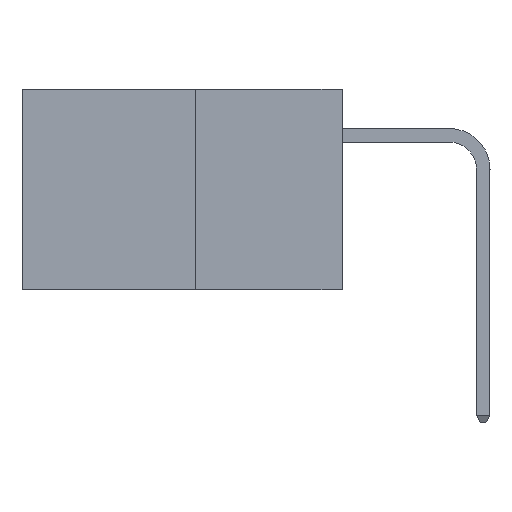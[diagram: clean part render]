
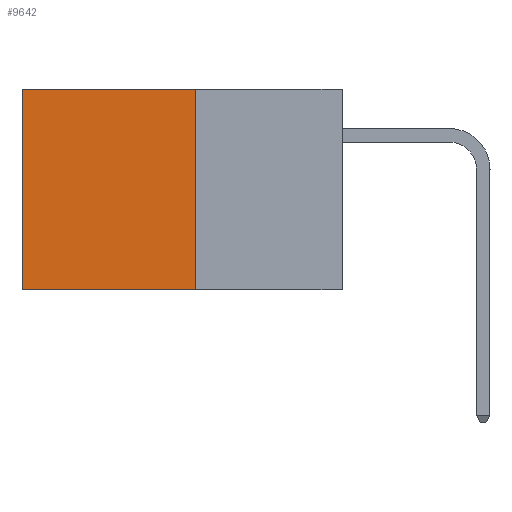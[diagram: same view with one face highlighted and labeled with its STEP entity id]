
A CAD part, left-side view. The second image highlights one B-rep face of the part: STEP entity #9642.
In plain terms, the highlighted planar face has unit normal (-1, 0, 0).
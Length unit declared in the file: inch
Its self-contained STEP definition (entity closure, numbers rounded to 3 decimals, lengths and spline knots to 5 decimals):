
#85 = CARTESIAN_POINT ( 'NONE',  ( 0.277, 0.27, 0. ) ) ;
#335 = DIRECTION ( 'NONE',  ( 0., 1., 0. ) ) ;
#445 = CARTESIAN_POINT ( 'NONE',  ( 0.277, 0.27, 0. ) ) ;
#870 = ORIENTED_EDGE ( 'NONE', *, *, #7032, .T. ) ;
#891 = CARTESIAN_POINT ( 'NONE',  ( 0.277, 0.27, -0.37 ) ) ;
#1509 = VECTOR ( 'NONE', #27543, 39.37008 ) ;
#1999 = AXIS2_PLACEMENT_3D ( 'NONE', #891, #3387, #20229 ) ;
#3387 = DIRECTION ( 'NONE',  ( 1., 0., 0. ) ) ;
#4537 = VECTOR ( 'NONE', #9559, 39.37008 ) ;
#5683 = ORIENTED_EDGE ( 'NONE', *, *, #7446, .F. ) ;
#6428 = VECTOR ( 'NONE', #335, 39.37008 ) ;
#7032 = EDGE_CURVE ( 'NONE', #19737, #27350, #27212, .T. ) ;
#7446 = EDGE_CURVE ( 'NONE', #8214, #23237, #7608, .T. ) ;
#7608 = LINE ( 'NONE', #17515, #13222 ) ;
#8106 = EDGE_CURVE ( 'NONE', #8214, #19737, #25670, .T. ) ;
#8214 = VERTEX_POINT ( 'NONE', #85 ) ;
#9559 = DIRECTION ( 'NONE',  ( 0., 1., 0. ) ) ;
#9642 = ADVANCED_FACE ( 'NONE', ( #23673 ), #15342, .F. ) ;
#13222 = VECTOR ( 'NONE', #17358, 39.37008 ) ;
#15241 = CARTESIAN_POINT ( 'NONE',  ( 0.277, 0.59, 0. ) ) ;
#15342 = PLANE ( 'NONE',  #1999 ) ;
#15514 = CARTESIAN_POINT ( 'NONE',  ( 0.277, 0.59, -0.37 ) ) ;
#17058 = ORIENTED_EDGE ( 'NONE', *, *, #23799, .F. ) ;
#17358 = DIRECTION ( 'NONE',  ( 0., 0., -1. ) ) ;
#17515 = CARTESIAN_POINT ( 'NONE',  ( 0.277, 0.27, -0.37 ) ) ;
#18848 = LINE ( 'NONE', #21587, #4537 ) ;
#19737 = VERTEX_POINT ( 'NONE', #15241 ) ;
#20229 = DIRECTION ( 'NONE',  ( 0., 0., -1. ) ) ;
#21587 = CARTESIAN_POINT ( 'NONE',  ( 0.277, 0.27, -0.37 ) ) ;
#23237 = VERTEX_POINT ( 'NONE', #30880 ) ;
#23673 = FACE_OUTER_BOUND ( 'NONE', #23804, .T. ) ;
#23799 = EDGE_CURVE ( 'NONE', #23237, #27350, #18848, .T. ) ;
#23804 = EDGE_LOOP ( 'NONE', ( #870, #17058, #5683, #26807 ) ) ;
#25670 = LINE ( 'NONE', #445, #6428 ) ;
#26807 = ORIENTED_EDGE ( 'NONE', *, *, #8106, .T. ) ;
#27212 = LINE ( 'NONE', #27477, #1509 ) ;
#27350 = VERTEX_POINT ( 'NONE', #15514 ) ;
#27477 = CARTESIAN_POINT ( 'NONE',  ( 0.277, 0.59, -0.37 ) ) ;
#27543 = DIRECTION ( 'NONE',  ( 0., 0., -1. ) ) ;
#30880 = CARTESIAN_POINT ( 'NONE',  ( 0.277, 0.27, -0.37 ) ) ;
